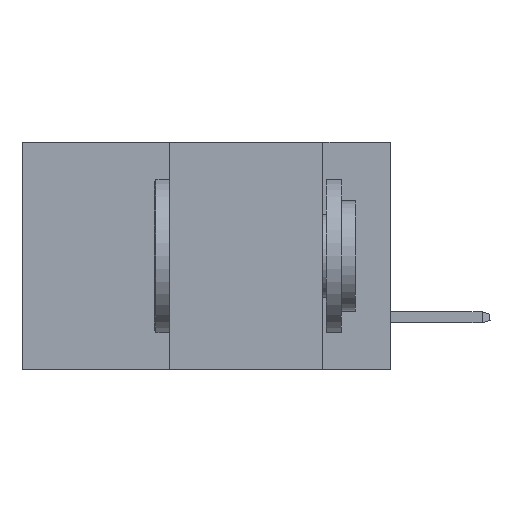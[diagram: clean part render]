
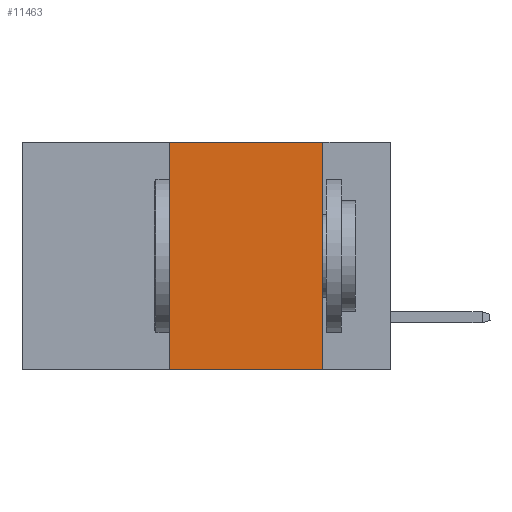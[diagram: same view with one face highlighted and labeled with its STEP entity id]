
A CAD part, left-side view. The second image highlights one B-rep face of the part: STEP entity #11463.
In plain terms, the highlighted planar face has unit normal (-1, 0, 0).
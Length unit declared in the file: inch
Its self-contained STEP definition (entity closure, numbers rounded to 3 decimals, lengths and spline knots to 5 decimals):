
#776 = ORIENTED_EDGE ( 'NONE', *, *, #20893, .F. ) ;
#1664 = FACE_OUTER_BOUND ( 'NONE', #34240, .T. ) ;
#1740 = VERTEX_POINT ( 'NONE', #35131 ) ;
#2766 = VECTOR ( 'NONE', #32062, 39.37008 ) ;
#2998 = AXIS2_PLACEMENT_3D ( 'NONE', #24098, #34966, #20035 ) ;
#3160 = EDGE_CURVE ( 'NONE', #1740, #30778, #36827, .T. ) ;
#3901 = CARTESIAN_POINT ( 'NONE',  ( 0., 0.11, -0.37 ) ) ;
#4869 = DIRECTION ( 'NONE',  ( 0., -1., 0. ) ) ;
#7727 = ORIENTED_EDGE ( 'NONE', *, *, #3160, .F. ) ;
#7851 = CARTESIAN_POINT ( 'NONE',  ( 0., 0.6, -0.37 ) ) ;
#7938 = CARTESIAN_POINT ( 'NONE',  ( 0., 0.36, -0.37 ) ) ;
#8994 = CARTESIAN_POINT ( 'NONE',  ( 0., 0.6, 0. ) ) ;
#11463 = ADVANCED_FACE ( 'NONE', ( #1664 ), #46018, .F. ) ;
#11685 = DIRECTION ( 'NONE',  ( 0., 0., 1. ) ) ;
#12461 = ORIENTED_EDGE ( 'NONE', *, *, #46564, .T. ) ;
#12805 = EDGE_CURVE ( 'NONE', #40673, #17266, #33889, .T. ) ;
#17266 = VERTEX_POINT ( 'NONE', #33491 ) ;
#20035 = DIRECTION ( 'NONE',  ( 0., 0., -1. ) ) ;
#20893 = EDGE_CURVE ( 'NONE', #17266, #1740, #44658, .T. ) ;
#21497 = CARTESIAN_POINT ( 'NONE',  ( 0., 0.36, 0. ) ) ;
#23267 = VECTOR ( 'NONE', #11685, 39.37008 ) ;
#24098 = CARTESIAN_POINT ( 'NONE',  ( 0., 0.6, 0. ) ) ;
#24714 = VECTOR ( 'NONE', #4869, 39.37008 ) ;
#26246 = DIRECTION ( 'NONE',  ( 0., -1., 0. ) ) ;
#27815 = LINE ( 'NONE', #7851, #48365 ) ;
#30778 = VERTEX_POINT ( 'NONE', #3901 ) ;
#32062 = DIRECTION ( 'NONE',  ( 0., 0., -1. ) ) ;
#33491 = CARTESIAN_POINT ( 'NONE',  ( 0., 0.36, 0. ) ) ;
#33889 = LINE ( 'NONE', #21497, #23267 ) ;
#34240 = EDGE_LOOP ( 'NONE', ( #7727, #776, #45302, #12461 ) ) ;
#34966 = DIRECTION ( 'NONE',  ( 1., 0., 0. ) ) ;
#35131 = CARTESIAN_POINT ( 'NONE',  ( 0., 0.11, 0. ) ) ;
#36827 = LINE ( 'NONE', #47721, #2766 ) ;
#40673 = VERTEX_POINT ( 'NONE', #7938 ) ;
#44658 = LINE ( 'NONE', #8994, #24714 ) ;
#45302 = ORIENTED_EDGE ( 'NONE', *, *, #12805, .F. ) ;
#46018 = PLANE ( 'NONE',  #2998 ) ;
#46564 = EDGE_CURVE ( 'NONE', #40673, #30778, #27815, .T. ) ;
#47721 = CARTESIAN_POINT ( 'NONE',  ( 0., 0.11, 0. ) ) ;
#48365 = VECTOR ( 'NONE', #26246, 39.37008 ) ;
